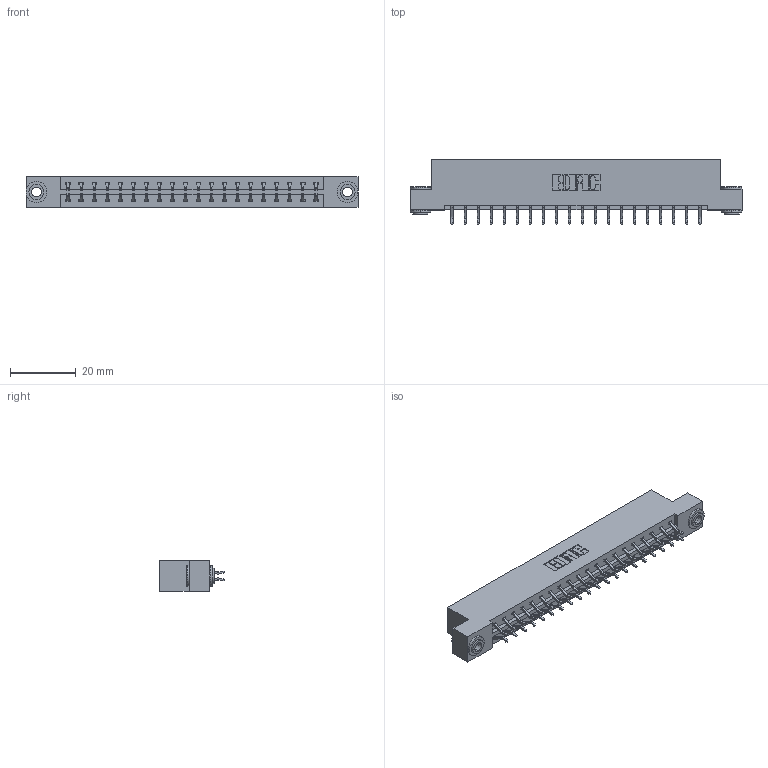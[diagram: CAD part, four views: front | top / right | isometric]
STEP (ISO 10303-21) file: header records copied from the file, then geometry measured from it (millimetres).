
FILE_DESCRIPTION (( 'STEP AP203' ), '1' );
FILE_NAME ('333-040-556-203.STEP', '2018-08-03T14:37:56', ( '' ), ( '' ), 'SwSTEP 2.0', 'SolidWorks 2016', '' );
FILE_SCHEMA (( 'CONFIG_CONTROL_DESIGN' ));
Length unit declared in the file: inch
Products named in the file (4): 345-250-002_345-250-002-102; 333-040-556-203; 333 Part_Flush - .156 Dia - TH; 345-292-001_556 Tail
Assembly tree (43 placements, depth 2):
  333-040-556-203
    333 Part_Flush - .156 Dia - TH
    345-292-001_556 Tail  x40
    345-250-002_345-250-002-102  x2
Bounding box: 100.79 x 19.57 x 9.4 mm (x, y, z)
Volume: 10101.9 mm3; surface area: 11888 mm2
Topology: 43 solids, 43 shells, 2472 faces, 7307 edges, 4814 vertices
Faces by surface type: plane 1680, cylinder 784, cone 8
Entity records: 16582 total; most frequent: CARTESIAN_POINT 2765, ORIENTED_EDGE 2682, DIRECTION 2423, EDGE_CURVE 1341, LINE 1181, VECTOR 1181, VERTEX_POINT 890, AXIS2_PLACEMENT_3D 621
